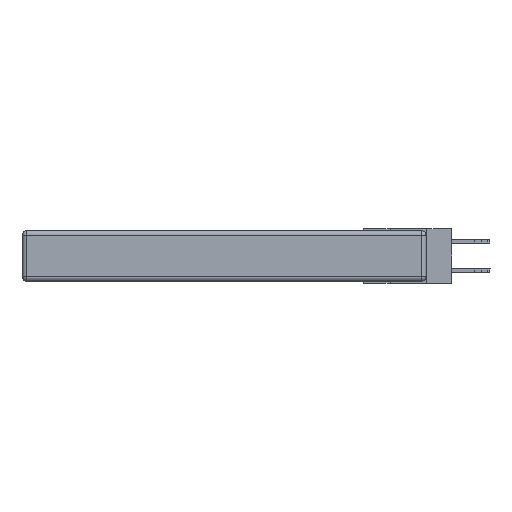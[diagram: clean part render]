
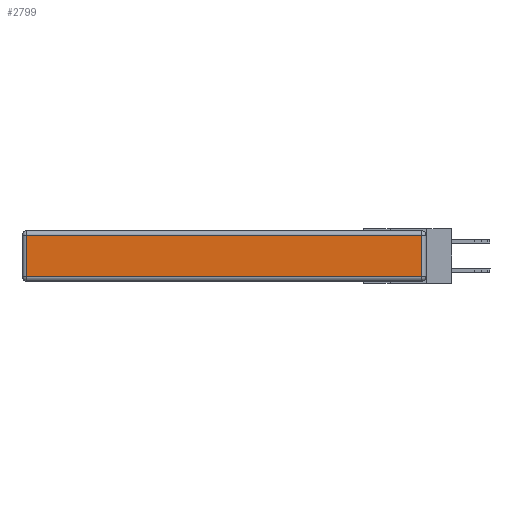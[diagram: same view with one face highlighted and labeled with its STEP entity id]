
A CAD part, left-side view. The second image highlights one B-rep face of the part: STEP entity #2799.
In plain terms, the highlighted planar face has unit normal (-1, 0, 0).
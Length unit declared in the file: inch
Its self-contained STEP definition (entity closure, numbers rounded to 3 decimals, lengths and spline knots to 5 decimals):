
#189 = DIRECTION ( 'NONE',  ( 0., 0., 1. ) ) ;
#1266 = CARTESIAN_POINT ( 'NONE',  ( 0., 2.72, -0.343 ) ) ;
#1558 = ORIENTED_EDGE ( 'NONE', *, *, #2080, .T. ) ;
#2080 = EDGE_CURVE ( 'NONE', #21239, #8869, #12035, .T. ) ;
#2555 = LINE ( 'NONE', #13122, #24394 ) ;
#2645 = AXIS2_PLACEMENT_3D ( 'NONE', #11071, #13352, #189 ) ;
#2799 = ADVANCED_FACE ( 'NONE', ( #7892 ), #8788, .T. ) ;
#4153 = VERTEX_POINT ( 'NONE', #13387 ) ;
#4465 = LINE ( 'NONE', #23599, #24954 ) ;
#5369 = EDGE_CURVE ( 'NONE', #23481, #4153, #4465, .T. ) ;
#7585 = VECTOR ( 'NONE', #18711, 39.37008 ) ;
#7892 = FACE_OUTER_BOUND ( 'NONE', #8635, .T. ) ;
#8553 = EDGE_CURVE ( 'NONE', #8869, #23481, #16144, .T. ) ;
#8635 = EDGE_LOOP ( 'NONE', ( #10468, #24672, #27246, #1558 ) ) ;
#8788 = PLANE ( 'NONE',  #2645 ) ;
#8869 = VERTEX_POINT ( 'NONE', #17437 ) ;
#10468 = ORIENTED_EDGE ( 'NONE', *, *, #8553, .T. ) ;
#11071 = CARTESIAN_POINT ( 'NONE',  ( 0., 0., -0.343 ) ) ;
#12035 = LINE ( 'NONE', #1266, #7585 ) ;
#12250 = CARTESIAN_POINT ( 'NONE',  ( 0., 0.03, -0.313 ) ) ;
#13122 = CARTESIAN_POINT ( 'NONE',  ( 0., 2.75, -0.03 ) ) ;
#13352 = DIRECTION ( 'NONE',  ( -1., 0., 0. ) ) ;
#13387 = CARTESIAN_POINT ( 'NONE',  ( 0., 0.03, -0.03 ) ) ;
#16144 = LINE ( 'NONE', #28150, #26771 ) ;
#16878 = EDGE_CURVE ( 'NONE', #4153, #21239, #2555, .T. ) ;
#17437 = CARTESIAN_POINT ( 'NONE',  ( 0., 2.72, -0.313 ) ) ;
#17468 = DIRECTION ( 'NONE',  ( 0., 0., 1. ) ) ;
#18711 = DIRECTION ( 'NONE',  ( 0., 0., -1. ) ) ;
#19257 = CARTESIAN_POINT ( 'NONE',  ( 0., 2.72, -0.03 ) ) ;
#21239 = VERTEX_POINT ( 'NONE', #19257 ) ;
#23481 = VERTEX_POINT ( 'NONE', #12250 ) ;
#23599 = CARTESIAN_POINT ( 'NONE',  ( 0., 0.03, -0.343 ) ) ;
#24394 = VECTOR ( 'NONE', #26202, 39.37008 ) ;
#24672 = ORIENTED_EDGE ( 'NONE', *, *, #5369, .T. ) ;
#24954 = VECTOR ( 'NONE', #17468, 39.37008 ) ;
#25934 = DIRECTION ( 'NONE',  ( 0., -1., 0. ) ) ;
#26202 = DIRECTION ( 'NONE',  ( 0., 1., 0. ) ) ;
#26771 = VECTOR ( 'NONE', #25934, 39.37008 ) ;
#27246 = ORIENTED_EDGE ( 'NONE', *, *, #16878, .T. ) ;
#28150 = CARTESIAN_POINT ( 'NONE',  ( 0., 0., -0.313 ) ) ;
